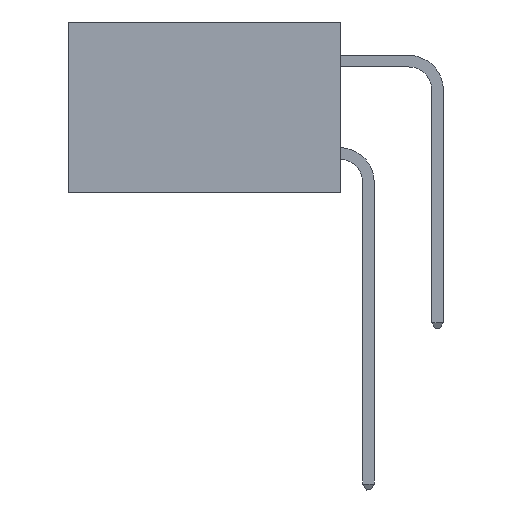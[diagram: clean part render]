
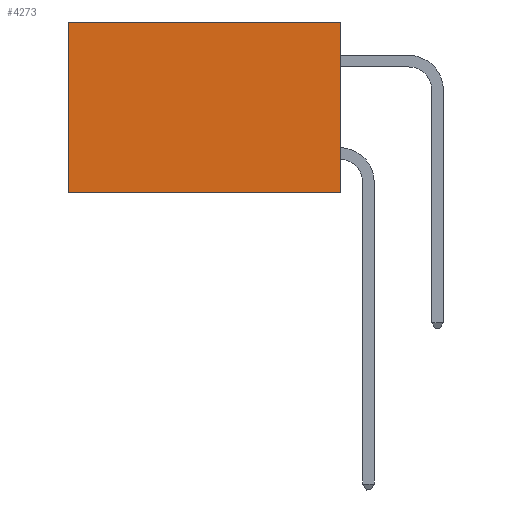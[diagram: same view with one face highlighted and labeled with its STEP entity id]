
A CAD part, left-side view. The second image highlights one B-rep face of the part: STEP entity #4273.
In plain terms, the highlighted planar face has unit normal (-1, 0, 0).
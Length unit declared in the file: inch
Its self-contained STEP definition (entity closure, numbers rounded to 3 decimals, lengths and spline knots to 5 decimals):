
#591 = EDGE_CURVE ( 'NONE', #4189, #8023, #1050, .T. ) ;
#938 = CARTESIAN_POINT ( 'NONE',  ( 0.277, 0.59, -0.37 ) ) ;
#946 = DIRECTION ( 'NONE',  ( 0., 0., -1. ) ) ;
#1050 = LINE ( 'NONE', #19005, #9319 ) ;
#1136 = FACE_OUTER_BOUND ( 'NONE', #10157, .T. ) ;
#1400 = VECTOR ( 'NONE', #946, 39.37008 ) ;
#1629 = AXIS2_PLACEMENT_3D ( 'NONE', #8473, #10050, #9993 ) ;
#4189 = VERTEX_POINT ( 'NONE', #13750 ) ;
#4273 = ADVANCED_FACE ( 'NONE', ( #1136 ), #10140, .F. ) ;
#5376 = CARTESIAN_POINT ( 'NONE',  ( 0.277, 0., 0. ) ) ;
#5633 = DIRECTION ( 'NONE',  ( 0., 1., 0. ) ) ;
#6813 = CARTESIAN_POINT ( 'NONE',  ( 0.277, 0., -0.37 ) ) ;
#7930 = LINE ( 'NONE', #10635, #11857 ) ;
#8023 = VERTEX_POINT ( 'NONE', #938 ) ;
#8473 = CARTESIAN_POINT ( 'NONE',  ( 0.277, 0., -0.37 ) ) ;
#9319 = VECTOR ( 'NONE', #9712, 39.37008 ) ;
#9712 = DIRECTION ( 'NONE',  ( 0., 0., -1. ) ) ;
#9993 = DIRECTION ( 'NONE',  ( 0., 0., -1. ) ) ;
#10050 = DIRECTION ( 'NONE',  ( 1., 0., 0. ) ) ;
#10140 = PLANE ( 'NONE',  #1629 ) ;
#10157 = EDGE_LOOP ( 'NONE', ( #17435, #16212, #16264, #16375 ) ) ;
#10635 = CARTESIAN_POINT ( 'NONE',  ( 0.277, 0., -0.37 ) ) ;
#11227 = VERTEX_POINT ( 'NONE', #6813 ) ;
#11857 = VECTOR ( 'NONE', #5633, 39.37008 ) ;
#11858 = EDGE_CURVE ( 'NONE', #13720, #4189, #14623, .T. ) ;
#12525 = CARTESIAN_POINT ( 'NONE',  ( 0.277, 0., -0.37 ) ) ;
#12650 = EDGE_CURVE ( 'NONE', #11227, #8023, #7930, .T. ) ;
#12706 = EDGE_CURVE ( 'NONE', #13720, #11227, #18638, .T. ) ;
#13720 = VERTEX_POINT ( 'NONE', #19371 ) ;
#13750 = CARTESIAN_POINT ( 'NONE',  ( 0.277, 0.59, 0. ) ) ;
#14623 = LINE ( 'NONE', #5376, #17739 ) ;
#16212 = ORIENTED_EDGE ( 'NONE', *, *, #12650, .F. ) ;
#16264 = ORIENTED_EDGE ( 'NONE', *, *, #12706, .F. ) ;
#16375 = ORIENTED_EDGE ( 'NONE', *, *, #11858, .T. ) ;
#17435 = ORIENTED_EDGE ( 'NONE', *, *, #591, .T. ) ;
#17739 = VECTOR ( 'NONE', #18203, 39.37008 ) ;
#18203 = DIRECTION ( 'NONE',  ( 0., 1., 0. ) ) ;
#18638 = LINE ( 'NONE', #12525, #1400 ) ;
#19005 = CARTESIAN_POINT ( 'NONE',  ( 0.277, 0.59, -0.37 ) ) ;
#19371 = CARTESIAN_POINT ( 'NONE',  ( 0.277, 0., 0. ) ) ;
